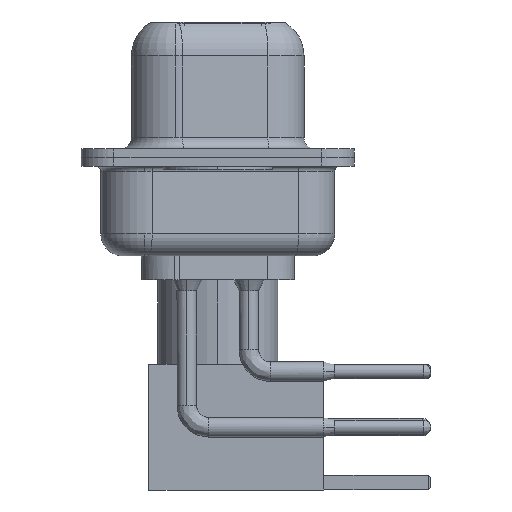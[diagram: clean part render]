
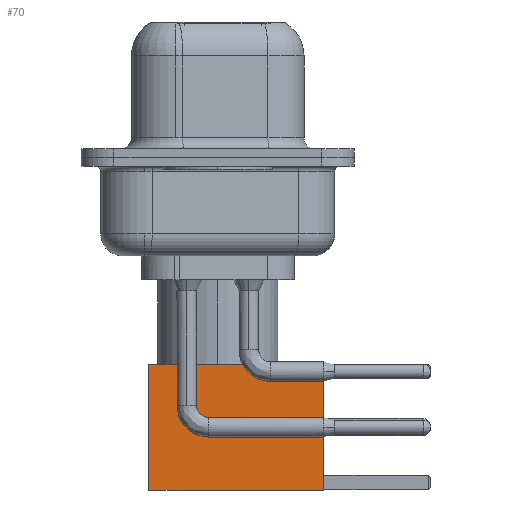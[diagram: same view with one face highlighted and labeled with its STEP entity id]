
A CAD part, left-side view. The second image highlights one B-rep face of the part: STEP entity #70.
In plain terms, the highlighted face is planar.
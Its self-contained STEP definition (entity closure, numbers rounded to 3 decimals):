
#70 = ADVANCED_FACE ( 'NONE', ( #15627 ), #1565, .T. ) ;
#1565 = PLANE ( 'NONE',  #11111 ) ;
#2340 = ORIENTED_EDGE ( 'NONE', *, *, #12049, .T. ) ;
#4277 = EDGE_CURVE ( 'NONE', #7333, #16766, #5902, .T. ) ;
#4306 = VECTOR ( 'NONE', #14247, 1000. ) ;
#4395 = CARTESIAN_POINT ( 'NONE',  ( -2.875, 2.875, 0. ) ) ;
#4498 = DIRECTION ( 'NONE',  ( 0., 0., 1. ) ) ;
#4527 = VECTOR ( 'NONE', #16712, 1000. ) ;
#4753 = CARTESIAN_POINT ( 'NONE',  ( 0., 2.875, 8. ) ) ;
#4987 = EDGE_LOOP ( 'NONE', ( #17363, #2340, #13253, #12411 ) ) ;
#5315 = EDGE_CURVE ( 'NONE', #12034, #7333, #6255, .T. ) ;
#5902 = LINE ( 'NONE', #4395, #6345 ) ;
#6255 = LINE ( 'NONE', #4753, #10625 ) ;
#6302 = DIRECTION ( 'NONE',  ( 0., 1., 0. ) ) ;
#6345 = VECTOR ( 'NONE', #19479, 1000. ) ;
#6485 = CARTESIAN_POINT ( 'NONE',  ( 2.875, 2.875, 0. ) ) ;
#7333 = VERTEX_POINT ( 'NONE', #19921 ) ;
#7468 = CARTESIAN_POINT ( 'NONE',  ( 2.875, 2.875, 8. ) ) ;
#9367 = CARTESIAN_POINT ( 'NONE',  ( 2.875, 2.875, 0. ) ) ;
#9892 = CARTESIAN_POINT ( 'NONE',  ( 0., 2.875, 0. ) ) ;
#10399 = CARTESIAN_POINT ( 'NONE',  ( -2.875, 2.875, 0. ) ) ;
#10558 = LINE ( 'NONE', #19951, #4527 ) ;
#10625 = VECTOR ( 'NONE', #11039, 1000. ) ;
#11039 = DIRECTION ( 'NONE',  ( -1., 0., 0. ) ) ;
#11111 = AXIS2_PLACEMENT_3D ( 'NONE', #9367, #6302, #4498 ) ;
#12034 = VERTEX_POINT ( 'NONE', #7468 ) ;
#12049 = EDGE_CURVE ( 'NONE', #18598, #16766, #15860, .T. ) ;
#12411 = ORIENTED_EDGE ( 'NONE', *, *, #5315, .F. ) ;
#13253 = ORIENTED_EDGE ( 'NONE', *, *, #4277, .F. ) ;
#14247 = DIRECTION ( 'NONE',  ( -1., 0., 0. ) ) ;
#15627 = FACE_OUTER_BOUND ( 'NONE', #4987, .T. ) ;
#15860 = LINE ( 'NONE', #9892, #4306 ) ;
#16712 = DIRECTION ( 'NONE',  ( 0., 0., -1. ) ) ;
#16766 = VERTEX_POINT ( 'NONE', #10399 ) ;
#17363 = ORIENTED_EDGE ( 'NONE', *, *, #18951, .T. ) ;
#18598 = VERTEX_POINT ( 'NONE', #6485 ) ;
#18951 = EDGE_CURVE ( 'NONE', #12034, #18598, #10558, .T. ) ;
#19479 = DIRECTION ( 'NONE',  ( 0., 0., -1. ) ) ;
#19921 = CARTESIAN_POINT ( 'NONE',  ( -2.875, 2.875, 8. ) ) ;
#19951 = CARTESIAN_POINT ( 'NONE',  ( 2.875, 2.875, 0. ) ) ;
